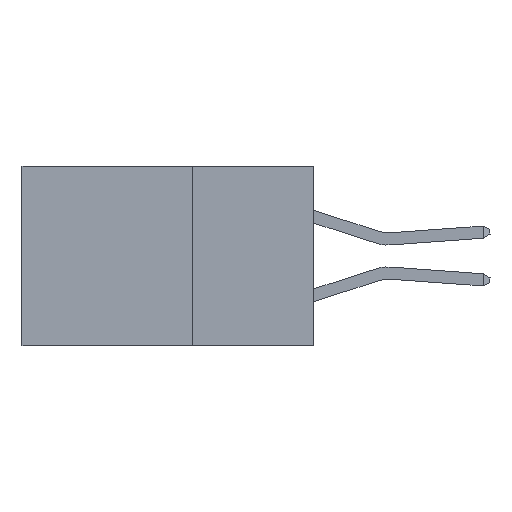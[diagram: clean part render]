
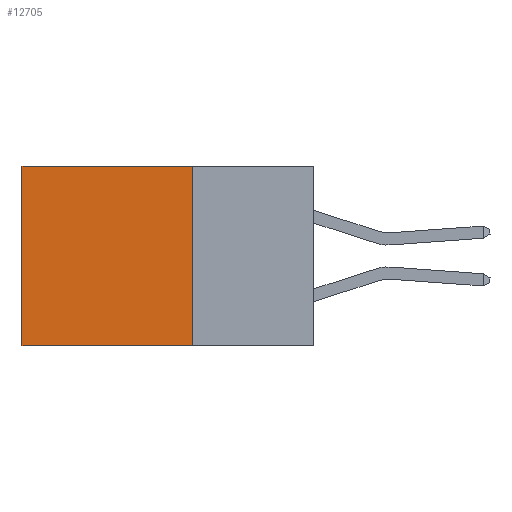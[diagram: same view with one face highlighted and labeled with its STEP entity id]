
A CAD part, left-side view. The second image highlights one B-rep face of the part: STEP entity #12705.
In plain terms, the highlighted planar face has unit normal (-1, 0, 0).
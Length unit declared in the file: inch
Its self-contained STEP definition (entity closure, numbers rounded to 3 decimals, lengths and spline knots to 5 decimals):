
#581 = EDGE_CURVE ( 'NONE', #37452, #37622, #7663, .T. ) ;
#1350 = CARTESIAN_POINT ( 'NONE',  ( 0.2875, 0.25, 0. ) ) ;
#1596 = CARTESIAN_POINT ( 'NONE',  ( 0.2875, 0.25, 0. ) ) ;
#1623 = DIRECTION ( 'NONE',  ( 0., 0., -1. ) ) ;
#2719 = ORIENTED_EDGE ( 'NONE', *, *, #23287, .F. ) ;
#3084 = ORIENTED_EDGE ( 'NONE', *, *, #581, .F. ) ;
#4016 = CARTESIAN_POINT ( 'NONE',  ( 0.2875, 0.25, 0. ) ) ;
#4917 = DIRECTION ( 'NONE',  ( 0., 1., 0. ) ) ;
#5491 = EDGE_CURVE ( 'NONE', #7004, #9538, #26975, .T. ) ;
#5513 = CARTESIAN_POINT ( 'NONE',  ( 0.2875, 0.6, -0.37 ) ) ;
#5762 = DIRECTION ( 'NONE',  ( 1., 0., 0. ) ) ;
#7004 = VERTEX_POINT ( 'NONE', #28139 ) ;
#7663 = LINE ( 'NONE', #1350, #20721 ) ;
#9538 = VERTEX_POINT ( 'NONE', #5513 ) ;
#9683 = LINE ( 'NONE', #24791, #25608 ) ;
#9982 = EDGE_CURVE ( 'NONE', #37452, #7004, #24961, .T. ) ;
#10188 = ORIENTED_EDGE ( 'NONE', *, *, #5491, .T. ) ;
#10842 = FACE_OUTER_BOUND ( 'NONE', #32272, .T. ) ;
#12705 = ADVANCED_FACE ( 'NONE', ( #10842 ), #20816, .F. ) ;
#14825 = DIRECTION ( 'NONE',  ( 0., 0., -1. ) ) ;
#16372 = DIRECTION ( 'NONE',  ( 0., 1., 0. ) ) ;
#17834 = AXIS2_PLACEMENT_3D ( 'NONE', #29928, #5762, #14825 ) ;
#20721 = VECTOR ( 'NONE', #1623, 39.37008 ) ;
#20816 = PLANE ( 'NONE',  #17834 ) ;
#21149 = ORIENTED_EDGE ( 'NONE', *, *, #9982, .T. ) ;
#23287 = EDGE_CURVE ( 'NONE', #37622, #9538, #9683, .T. ) ;
#24042 = DIRECTION ( 'NONE',  ( 0., 0., -1. ) ) ;
#24791 = CARTESIAN_POINT ( 'NONE',  ( 0.2875, 0.25, -0.37 ) ) ;
#24961 = LINE ( 'NONE', #1596, #36255 ) ;
#25608 = VECTOR ( 'NONE', #16372, 39.37008 ) ;
#26573 = CARTESIAN_POINT ( 'NONE',  ( 0.2875, 0.6, 0. ) ) ;
#26975 = LINE ( 'NONE', #26573, #29830 ) ;
#28139 = CARTESIAN_POINT ( 'NONE',  ( 0.2875, 0.6, 0. ) ) ;
#28974 = CARTESIAN_POINT ( 'NONE',  ( 0.2875, 0.25, -0.37 ) ) ;
#29830 = VECTOR ( 'NONE', #24042, 39.37008 ) ;
#29928 = CARTESIAN_POINT ( 'NONE',  ( 0.2875, 0.25, 0. ) ) ;
#32272 = EDGE_LOOP ( 'NONE', ( #10188, #2719, #3084, #21149 ) ) ;
#36255 = VECTOR ( 'NONE', #4917, 39.37008 ) ;
#37452 = VERTEX_POINT ( 'NONE', #4016 ) ;
#37622 = VERTEX_POINT ( 'NONE', #28974 ) ;
